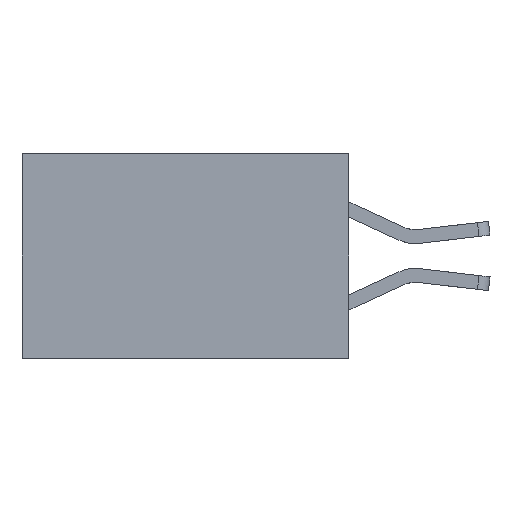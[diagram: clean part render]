
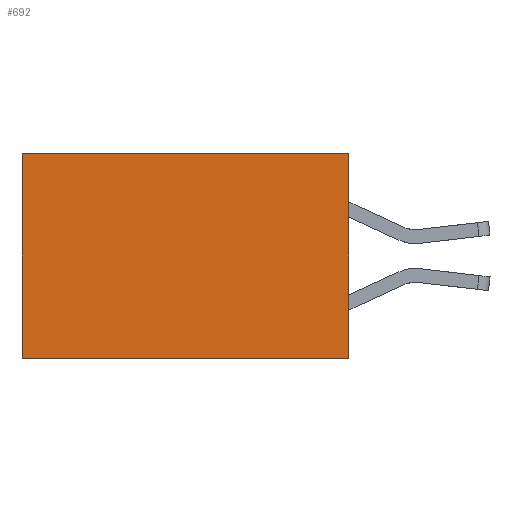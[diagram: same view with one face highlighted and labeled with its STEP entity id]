
A CAD part, left-side view. The second image highlights one B-rep face of the part: STEP entity #692.
In plain terms, the highlighted planar face has unit normal (-1, 0, 0).
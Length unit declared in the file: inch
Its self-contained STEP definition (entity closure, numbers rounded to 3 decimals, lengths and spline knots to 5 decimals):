
#107 = CARTESIAN_POINT ( 'NONE',  ( 0.277, 0.59, -0.37 ) ) ;
#122 = DIRECTION ( 'NONE',  ( 0., 0., -1. ) ) ;
#308 = EDGE_LOOP ( 'NONE', ( #6676, #1727, #816, #863 ) ) ;
#510 = DIRECTION ( 'NONE',  ( 0., 1., 0. ) ) ;
#692 = ADVANCED_FACE ( 'NONE', ( #10152 ), #8529, .F. ) ;
#718 = LINE ( 'NONE', #2769, #6194 ) ;
#816 = ORIENTED_EDGE ( 'NONE', *, *, #4374, .F. ) ;
#863 = ORIENTED_EDGE ( 'NONE', *, *, #11056, .T. ) ;
#1255 = VECTOR ( 'NONE', #8631, 39.37008 ) ;
#1670 = VERTEX_POINT ( 'NONE', #10819 ) ;
#1727 = ORIENTED_EDGE ( 'NONE', *, *, #12260, .F. ) ;
#2067 = LINE ( 'NONE', #7048, #2438 ) ;
#2438 = VECTOR ( 'NONE', #510, 39.37008 ) ;
#2547 = LINE ( 'NONE', #107, #13797 ) ;
#2769 = CARTESIAN_POINT ( 'NONE',  ( 0.277, 0., 0. ) ) ;
#3635 = VERTEX_POINT ( 'NONE', #6508 ) ;
#3846 = DIRECTION ( 'NONE',  ( 0., 1., 0. ) ) ;
#4150 = LINE ( 'NONE', #9994, #1255 ) ;
#4374 = EDGE_CURVE ( 'NONE', #13694, #3635, #4150, .T. ) ;
#6002 = AXIS2_PLACEMENT_3D ( 'NONE', #6898, #8696, #11566 ) ;
#6194 = VECTOR ( 'NONE', #3846, 39.37008 ) ;
#6508 = CARTESIAN_POINT ( 'NONE',  ( 0.277, 0., -0.37 ) ) ;
#6676 = ORIENTED_EDGE ( 'NONE', *, *, #8398, .T. ) ;
#6898 = CARTESIAN_POINT ( 'NONE',  ( 0.277, 0., -0.37 ) ) ;
#7048 = CARTESIAN_POINT ( 'NONE',  ( 0.277, 0., -0.37 ) ) ;
#8398 = EDGE_CURVE ( 'NONE', #1670, #10078, #2547, .T. ) ;
#8529 = PLANE ( 'NONE',  #6002 ) ;
#8631 = DIRECTION ( 'NONE',  ( 0., 0., -1. ) ) ;
#8696 = DIRECTION ( 'NONE',  ( 1., 0., 0. ) ) ;
#9718 = CARTESIAN_POINT ( 'NONE',  ( 0.277, 0.59, -0.37 ) ) ;
#9994 = CARTESIAN_POINT ( 'NONE',  ( 0.277, 0., -0.37 ) ) ;
#10078 = VERTEX_POINT ( 'NONE', #9718 ) ;
#10152 = FACE_OUTER_BOUND ( 'NONE', #308, .T. ) ;
#10819 = CARTESIAN_POINT ( 'NONE',  ( 0.277, 0.59, 0. ) ) ;
#11056 = EDGE_CURVE ( 'NONE', #13694, #1670, #718, .T. ) ;
#11566 = DIRECTION ( 'NONE',  ( 0., 0., -1. ) ) ;
#12260 = EDGE_CURVE ( 'NONE', #3635, #10078, #2067, .T. ) ;
#13694 = VERTEX_POINT ( 'NONE', #14069 ) ;
#13797 = VECTOR ( 'NONE', #122, 39.37008 ) ;
#14069 = CARTESIAN_POINT ( 'NONE',  ( 0.277, 0., 0. ) ) ;
